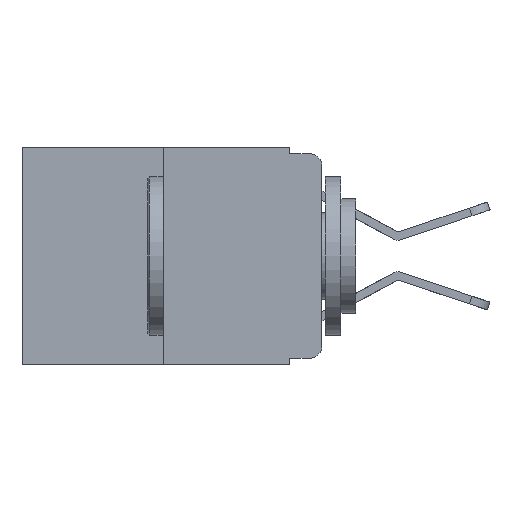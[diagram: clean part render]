
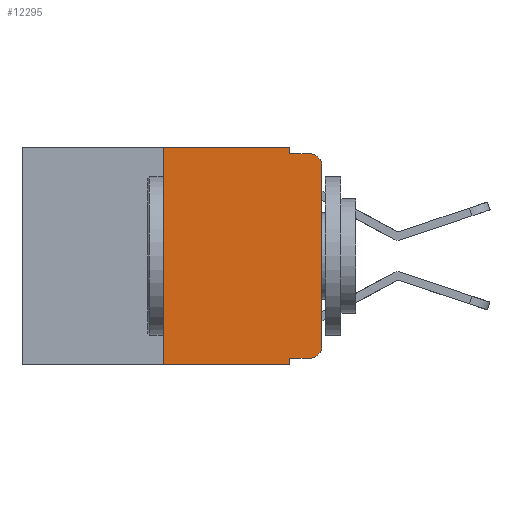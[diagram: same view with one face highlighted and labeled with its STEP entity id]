
A CAD part, left-side view. The second image highlights one B-rep face of the part: STEP entity #12295.
In plain terms, the highlighted planar face has unit normal (-1, 0, 0).
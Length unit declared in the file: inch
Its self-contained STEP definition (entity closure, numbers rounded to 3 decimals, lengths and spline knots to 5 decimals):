
#796 = DIRECTION ( 'NONE',  ( 0., 0., -1. ) ) ;
#938 = CARTESIAN_POINT ( 'NONE',  ( 0., 0., -0.03 ) ) ;
#1157 = LINE ( 'NONE', #6707, #5371 ) ;
#1401 = LINE ( 'NONE', #2170, #16419 ) ;
#1526 = DIRECTION ( 'NONE',  ( 0., 0., -1. ) ) ;
#1717 = VECTOR ( 'NONE', #4869, 39.37008 ) ;
#1974 = CARTESIAN_POINT ( 'NONE',  ( 0., 0.473, 0. ) ) ;
#2148 = VERTEX_POINT ( 'NONE', #15083 ) ;
#2170 = CARTESIAN_POINT ( 'NONE',  ( 0., 0.25, 0. ) ) ;
#2295 = ORIENTED_EDGE ( 'NONE', *, *, #18754, .F. ) ;
#2585 = PLANE ( 'NONE',  #16481 ) ;
#2842 = EDGE_CURVE ( 'NONE', #9596, #2148, #14471, .T. ) ;
#2987 = CARTESIAN_POINT ( 'NONE',  ( 0., 0.02, -0.333 ) ) ;
#3178 = VERTEX_POINT ( 'NONE', #2987 ) ;
#3259 = ORIENTED_EDGE ( 'NONE', *, *, #5295, .T. ) ;
#3798 = CARTESIAN_POINT ( 'NONE',  ( 0., 0.051, 0. ) ) ;
#4091 = DIRECTION ( 'NONE',  ( 0., -1., 0. ) ) ;
#4167 = VECTOR ( 'NONE', #4091, 39.37008 ) ;
#4290 = DIRECTION ( 'NONE',  ( 0., 0., 1. ) ) ;
#4869 = DIRECTION ( 'NONE',  ( 0., 0., 1. ) ) ;
#5027 = CARTESIAN_POINT ( 'NONE',  ( 0., 0.02, -0.01 ) ) ;
#5295 = EDGE_CURVE ( 'NONE', #19778, #14183, #17907, .T. ) ;
#5371 = VECTOR ( 'NONE', #18132, 39.37008 ) ;
#5672 = DIRECTION ( 'NONE',  ( 0., 0., -1. ) ) ;
#6396 = ORIENTED_EDGE ( 'NONE', *, *, #15829, .T. ) ;
#6572 = VERTEX_POINT ( 'NONE', #11927 ) ;
#6707 = CARTESIAN_POINT ( 'NONE',  ( 0., 0.473, -0.343 ) ) ;
#7026 = ORIENTED_EDGE ( 'NONE', *, *, #12943, .T. ) ;
#7092 = CARTESIAN_POINT ( 'NONE',  ( 0., 0.051, -0.333 ) ) ;
#7965 = LINE ( 'NONE', #7092, #16812 ) ;
#8820 = ORIENTED_EDGE ( 'NONE', *, *, #12064, .F. ) ;
#9418 = VECTOR ( 'NONE', #5672, 39.37008 ) ;
#9567 = CARTESIAN_POINT ( 'NONE',  ( 0., 0., 0. ) ) ;
#9568 = CARTESIAN_POINT ( 'NONE',  ( 0., 0., -0.313 ) ) ;
#9596 = VERTEX_POINT ( 'NONE', #23755 ) ;
#9736 = EDGE_CURVE ( 'NONE', #20017, #23442, #10453, .T. ) ;
#10074 = CARTESIAN_POINT ( 'NONE',  ( 0., 0.25, -0.343 ) ) ;
#10226 = DIRECTION ( 'NONE',  ( -1., 0., 0. ) ) ;
#10453 = LINE ( 'NONE', #24076, #24933 ) ;
#10755 = DIRECTION ( 'NONE',  ( 0., 0., -1. ) ) ;
#11560 = CARTESIAN_POINT ( 'NONE',  ( 0., 0.051, -0.01 ) ) ;
#11927 = CARTESIAN_POINT ( 'NONE',  ( 0., 0.25, 0. ) ) ;
#12000 = LINE ( 'NONE', #11560, #16309 ) ;
#12064 = EDGE_CURVE ( 'NONE', #6572, #20017, #14531, .T. ) ;
#12226 = EDGE_CURVE ( 'NONE', #23442, #23022, #12000, .T. ) ;
#12295 = ADVANCED_FACE ( 'NONE', ( #24839 ), #2585, .F. ) ;
#12408 = EDGE_CURVE ( 'NONE', #9596, #3178, #7965, .T. ) ;
#12816 = ORIENTED_EDGE ( 'NONE', *, *, #2842, .F. ) ;
#12943 = EDGE_CURVE ( 'NONE', #23260, #2148, #1157, .T. ) ;
#13471 = DIRECTION ( 'NONE',  ( -1., 0., 0. ) ) ;
#13632 = ORIENTED_EDGE ( 'NONE', *, *, #12226, .F. ) ;
#14183 = VERTEX_POINT ( 'NONE', #938 ) ;
#14471 = LINE ( 'NONE', #3798, #9418 ) ;
#14531 = LINE ( 'NONE', #1974, #4167 ) ;
#15025 = AXIS2_PLACEMENT_3D ( 'NONE', #24723, #13471, #1526 ) ;
#15083 = CARTESIAN_POINT ( 'NONE',  ( 0., 0.051, -0.343 ) ) ;
#15829 = EDGE_CURVE ( 'NONE', #14183, #23022, #18636, .T. ) ;
#16309 = VECTOR ( 'NONE', #24739, 39.37008 ) ;
#16419 = VECTOR ( 'NONE', #4290, 39.37008 ) ;
#16481 = AXIS2_PLACEMENT_3D ( 'NONE', #18240, #22042, #10755 ) ;
#16812 = VECTOR ( 'NONE', #24111, 39.37008 ) ;
#17722 = CARTESIAN_POINT ( 'NONE',  ( 0., 0.051, 0. ) ) ;
#17907 = LINE ( 'NONE', #9567, #1717 ) ;
#18102 = ORIENTED_EDGE ( 'NONE', *, *, #12408, .T. ) ;
#18132 = DIRECTION ( 'NONE',  ( 0., -1., 0. ) ) ;
#18240 = CARTESIAN_POINT ( 'NONE',  ( 0., 0.473, 0. ) ) ;
#18636 = CIRCLE ( 'NONE', #15025, 0.02 ) ;
#18754 = EDGE_CURVE ( 'NONE', #23260, #6572, #1401, .T. ) ;
#19197 = ORIENTED_EDGE ( 'NONE', *, *, #22643, .T. ) ;
#19778 = VERTEX_POINT ( 'NONE', #9568 ) ;
#20017 = VERTEX_POINT ( 'NONE', #17722 ) ;
#21510 = CARTESIAN_POINT ( 'NONE',  ( 0., 0.02, -0.313 ) ) ;
#21911 = AXIS2_PLACEMENT_3D ( 'NONE', #21510, #10226, #23434 ) ;
#21937 = CARTESIAN_POINT ( 'NONE',  ( 0., 0.051, -0.01 ) ) ;
#22042 = DIRECTION ( 'NONE',  ( 1., 0., 0. ) ) ;
#22619 = ORIENTED_EDGE ( 'NONE', *, *, #9736, .F. ) ;
#22643 = EDGE_CURVE ( 'NONE', #3178, #19778, #25041, .T. ) ;
#23022 = VERTEX_POINT ( 'NONE', #5027 ) ;
#23260 = VERTEX_POINT ( 'NONE', #10074 ) ;
#23434 = DIRECTION ( 'NONE',  ( 0., 0., -1. ) ) ;
#23442 = VERTEX_POINT ( 'NONE', #21937 ) ;
#23755 = CARTESIAN_POINT ( 'NONE',  ( 0., 0.051, -0.333 ) ) ;
#24076 = CARTESIAN_POINT ( 'NONE',  ( 0., 0.051, 0. ) ) ;
#24111 = DIRECTION ( 'NONE',  ( 0., -1., 0. ) ) ;
#24171 = EDGE_LOOP ( 'NONE', ( #3259, #6396, #13632, #22619, #8820, #2295, #7026, #12816, #18102, #19197 ) ) ;
#24723 = CARTESIAN_POINT ( 'NONE',  ( 0., 0.02, -0.03 ) ) ;
#24739 = DIRECTION ( 'NONE',  ( 0., -1., 0. ) ) ;
#24839 = FACE_OUTER_BOUND ( 'NONE', #24171, .T. ) ;
#24933 = VECTOR ( 'NONE', #796, 39.37008 ) ;
#25041 = CIRCLE ( 'NONE', #21911, 0.02 ) ;
